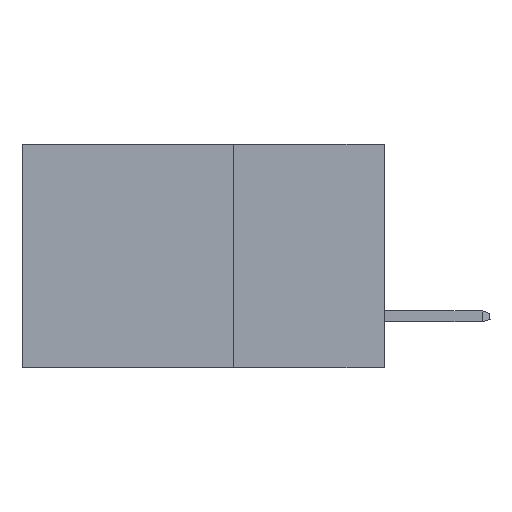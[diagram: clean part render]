
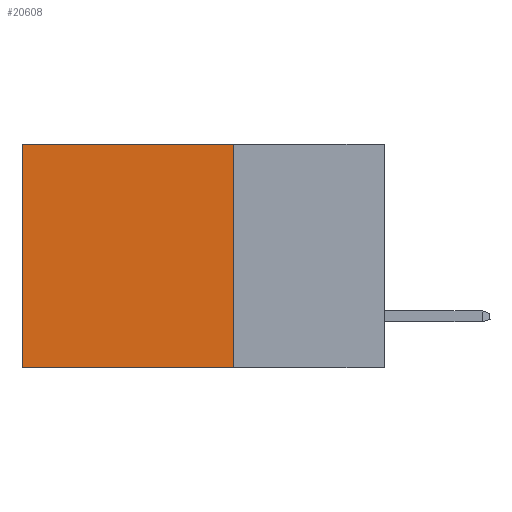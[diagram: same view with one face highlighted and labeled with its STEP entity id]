
A CAD part, left-side view. The second image highlights one B-rep face of the part: STEP entity #20608.
In plain terms, the highlighted planar face has unit normal (-1, 0, 0).
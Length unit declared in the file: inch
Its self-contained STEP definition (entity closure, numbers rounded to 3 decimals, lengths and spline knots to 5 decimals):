
#509 = VERTEX_POINT ( 'NONE', #18748 ) ;
#844 = DIRECTION ( 'NONE',  ( 1., 0., 0. ) ) ;
#911 = CARTESIAN_POINT ( 'NONE',  ( 0.298, 0.25, 0. ) ) ;
#1051 = ORIENTED_EDGE ( 'NONE', *, *, #12360, .F. ) ;
#1620 = EDGE_CURVE ( 'NONE', #509, #19609, #21282, .T. ) ;
#3381 = CARTESIAN_POINT ( 'NONE',  ( 0.298, 0.25, -0.37 ) ) ;
#3432 = VECTOR ( 'NONE', #19489, 39.37008 ) ;
#3706 = VECTOR ( 'NONE', #26001, 39.37008 ) ;
#4969 = EDGE_LOOP ( 'NONE', ( #7259, #28824, #1051, #26143 ) ) ;
#6097 = AXIS2_PLACEMENT_3D ( 'NONE', #14688, #844, #17051 ) ;
#6386 = CARTESIAN_POINT ( 'NONE',  ( 0.298, 0.25, -0.37 ) ) ;
#6425 = VECTOR ( 'NONE', #24328, 39.37008 ) ;
#7259 = ORIENTED_EDGE ( 'NONE', *, *, #26512, .T. ) ;
#7976 = CARTESIAN_POINT ( 'NONE',  ( 0.298, 0.6, -0.37 ) ) ;
#9704 = FACE_OUTER_BOUND ( 'NONE', #4969, .T. ) ;
#10449 = CARTESIAN_POINT ( 'NONE',  ( 0.298, 0.25, 0. ) ) ;
#11265 = VECTOR ( 'NONE', #17416, 39.37008 ) ;
#12138 = VERTEX_POINT ( 'NONE', #6386 ) ;
#12360 = EDGE_CURVE ( 'NONE', #509, #12138, #18163, .T. ) ;
#12884 = VERTEX_POINT ( 'NONE', #7976 ) ;
#14688 = CARTESIAN_POINT ( 'NONE',  ( 0.298, 0.25, 0. ) ) ;
#17051 = DIRECTION ( 'NONE',  ( 0., 0., -1. ) ) ;
#17416 = DIRECTION ( 'NONE',  ( 0., 0., -1. ) ) ;
#17494 = LINE ( 'NONE', #23673, #3706 ) ;
#18163 = LINE ( 'NONE', #10449, #11265 ) ;
#18748 = CARTESIAN_POINT ( 'NONE',  ( 0.298, 0.25, 0. ) ) ;
#19489 = DIRECTION ( 'NONE',  ( 0., 1., 0. ) ) ;
#19609 = VERTEX_POINT ( 'NONE', #29884 ) ;
#20608 = ADVANCED_FACE ( 'NONE', ( #9704 ), #26315, .F. ) ;
#21282 = LINE ( 'NONE', #911, #3432 ) ;
#23673 = CARTESIAN_POINT ( 'NONE',  ( 0.298, 0.6, 0. ) ) ;
#24328 = DIRECTION ( 'NONE',  ( 0., 1., 0. ) ) ;
#25708 = LINE ( 'NONE', #3381, #6425 ) ;
#26001 = DIRECTION ( 'NONE',  ( 0., 0., -1. ) ) ;
#26143 = ORIENTED_EDGE ( 'NONE', *, *, #1620, .T. ) ;
#26315 = PLANE ( 'NONE',  #6097 ) ;
#26512 = EDGE_CURVE ( 'NONE', #19609, #12884, #17494, .T. ) ;
#28824 = ORIENTED_EDGE ( 'NONE', *, *, #29613, .F. ) ;
#29613 = EDGE_CURVE ( 'NONE', #12138, #12884, #25708, .T. ) ;
#29884 = CARTESIAN_POINT ( 'NONE',  ( 0.298, 0.6, 0. ) ) ;
